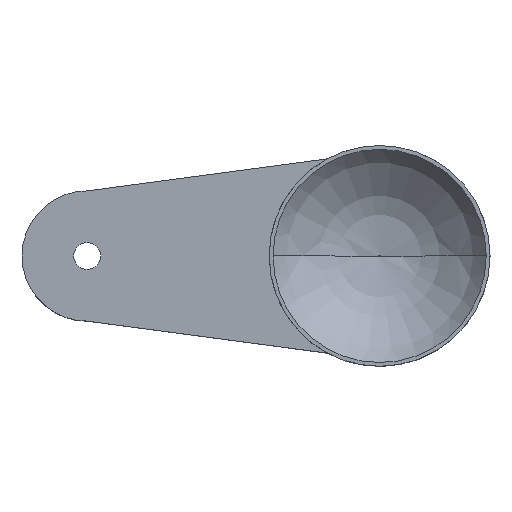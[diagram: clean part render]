
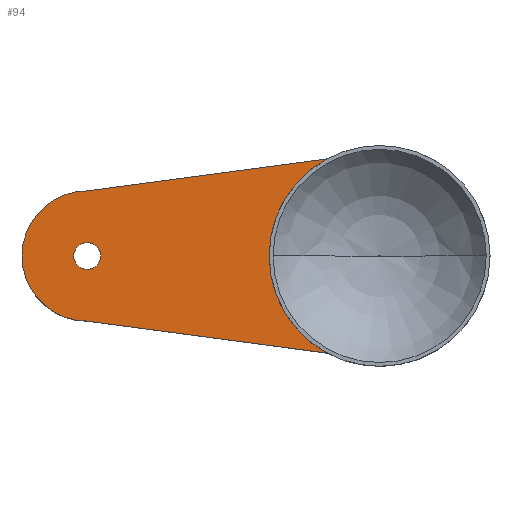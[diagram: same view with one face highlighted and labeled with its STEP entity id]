
A CAD part, top view. The second image highlights one B-rep face of the part: STEP entity #94.
In plain terms, the highlighted planar face has unit normal (0, 0, 1).
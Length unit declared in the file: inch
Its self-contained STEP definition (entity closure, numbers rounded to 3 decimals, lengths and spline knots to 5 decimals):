
#6 = LINE ( 'NONE', #535, #542 ) ;
#8 = EDGE_CURVE ( 'NONE', #490, #29, #429, .T. ) ;
#10 = DIRECTION ( 'NONE',  ( 0.991, 0.132, 0. ) ) ;
#24 = AXIS2_PLACEMENT_3D ( 'NONE', #163, #158, #155 ) ;
#29 = VERTEX_POINT ( 'NONE', #306 ) ;
#41 = DIRECTION ( 'NONE',  ( 1., 0., 0. ) ) ;
#43 = DIRECTION ( 'NONE',  ( 0., 0., 1. ) ) ;
#44 = AXIS2_PLACEMENT_3D ( 'NONE', #70, #43, #41 ) ;
#49 = EDGE_CURVE ( 'NONE', #430, #426, #289, .T. ) ;
#59 = ORIENTED_EDGE ( 'NONE', *, *, #267, .T. ) ;
#63 = CARTESIAN_POINT ( 'NONE',  ( 23.73897, 25.66022, 4. ) ) ;
#64 = CIRCLE ( 'NONE', #520, 2.43417 ) ;
#67 = CARTESIAN_POINT ( 'NONE',  ( -3.38477, 25.38511, 4. ) ) ;
#70 = CARTESIAN_POINT ( 'NONE',  ( 16.93431, 25.66022, 4. ) ) ;
#77 = ORIENTED_EDGE ( 'NONE', *, *, #460, .F. ) ;
#82 = DIRECTION ( 'NONE',  ( 1., 0., 0. ) ) ;
#85 = VECTOR ( 'NONE', #10, 39.37008 ) ;
#94 = ADVANCED_FACE ( 'NONE', ( #146, #557 ), #541, .T. ) ;
#99 = ORIENTED_EDGE ( 'NONE', *, *, #493, .F. ) ;
#146 = FACE_OUTER_BOUND ( 'NONE', #414, .T. ) ;
#155 = DIRECTION ( 'NONE',  ( 1., 0., 0. ) ) ;
#158 = DIRECTION ( 'NONE',  ( 0., 0., 1. ) ) ;
#160 = CARTESIAN_POINT ( 'NONE',  ( 16.93431, 23.22605, 4. ) ) ;
#163 = CARTESIAN_POINT ( 'NONE',  ( 27.86307, 25.66022, 4. ) ) ;
#171 = DIRECTION ( 'NONE',  ( 0., 0., 1. ) ) ;
#180 = CARTESIAN_POINT ( 'NONE',  ( 16.93431, 25.66022, 4. ) ) ;
#182 = EDGE_CURVE ( 'NONE', #317, #29, #6, .T. ) ;
#214 = ORIENTED_EDGE ( 'NONE', *, *, #539, .F. ) ;
#219 = LINE ( 'NONE', #67, #85 ) ;
#224 = DIRECTION ( 'NONE',  ( 0., 0., 1. ) ) ;
#229 = ORIENTED_EDGE ( 'NONE', *, *, #547, .T. ) ;
#260 = CARTESIAN_POINT ( 'NONE',  ( 25.90666, 29.29074, 4. ) ) ;
#267 = EDGE_CURVE ( 'NONE', #583, #317, #563, .T. ) ;
#289 = CIRCLE ( 'NONE', #417, 0.50198 ) ;
#306 = CARTESIAN_POINT ( 'NONE',  ( 25.90666, 22.0297, 4. ) ) ;
#317 = VERTEX_POINT ( 'NONE', #160 ) ;
#318 = CARTESIAN_POINT ( 'NONE',  ( 17.43629, 25.66022, 4. ) ) ;
#326 = AXIS2_PLACEMENT_3D ( 'NONE', #498, #560, #452 ) ;
#334 = ORIENTED_EDGE ( 'NONE', *, *, #182, .T. ) ;
#351 = VERTEX_POINT ( 'NONE', #260 ) ;
#399 = VERTEX_POINT ( 'NONE', #527 ) ;
#414 = EDGE_LOOP ( 'NONE', ( #99, #229, #59, #334, #606, #77 ) ) ;
#417 = AXIS2_PLACEMENT_3D ( 'NONE', #653, #650, #649 ) ;
#426 = VERTEX_POINT ( 'NONE', #489 ) ;
#429 = CIRCLE ( 'NONE', #445, 4.1241 ) ;
#430 = VERTEX_POINT ( 'NONE', #318 ) ;
#445 = AXIS2_PLACEMENT_3D ( 'NONE', #631, #224, #637 ) ;
#452 = DIRECTION ( 'NONE',  ( 1., 0., 0. ) ) ;
#454 = ORIENTED_EDGE ( 'NONE', *, *, #49, .F. ) ;
#460 = EDGE_CURVE ( 'NONE', #351, #490, #599, .T. ) ;
#468 = CIRCLE ( 'NONE', #524, 0.50198 ) ;
#489 = CARTESIAN_POINT ( 'NONE',  ( 16.43233, 25.66022, 4. ) ) ;
#490 = VERTEX_POINT ( 'NONE', #63 ) ;
#493 = EDGE_CURVE ( 'NONE', #399, #351, #219, .T. ) ;
#497 = CARTESIAN_POINT ( 'NONE',  ( 14.50013, 25.66022, 4. ) ) ;
#498 = CARTESIAN_POINT ( 'NONE',  ( 0., 0., 4. ) ) ;
#501 = DIRECTION ( 'NONE',  ( 0.991, -0.132, 0. ) ) ;
#520 = AXIS2_PLACEMENT_3D ( 'NONE', #639, #636, #630 ) ;
#524 = AXIS2_PLACEMENT_3D ( 'NONE', #180, #171, #82 ) ;
#527 = CARTESIAN_POINT ( 'NONE',  ( 16.93431, 28.09439, 4. ) ) ;
#535 = CARTESIAN_POINT ( 'NONE',  ( 3.3386, 25.03885, 4. ) ) ;
#539 = EDGE_CURVE ( 'NONE', #426, #430, #468, .T. ) ;
#541 = PLANE ( 'NONE',  #326 ) ;
#542 = VECTOR ( 'NONE', #501, 39.37008 ) ;
#547 = EDGE_CURVE ( 'NONE', #399, #583, #64, .T. ) ;
#557 = FACE_BOUND ( 'NONE', #594, .T. ) ;
#560 = DIRECTION ( 'NONE',  ( 0., 0., 1. ) ) ;
#563 = CIRCLE ( 'NONE', #44, 2.43417 ) ;
#583 = VERTEX_POINT ( 'NONE', #497 ) ;
#594 = EDGE_LOOP ( 'NONE', ( #214, #454 ) ) ;
#599 = CIRCLE ( 'NONE', #24, 4.1241 ) ;
#606 = ORIENTED_EDGE ( 'NONE', *, *, #8, .F. ) ;
#630 = DIRECTION ( 'NONE',  ( 1., 0., 0. ) ) ;
#631 = CARTESIAN_POINT ( 'NONE',  ( 27.86307, 25.66022, 4. ) ) ;
#636 = DIRECTION ( 'NONE',  ( 0., 0., 1. ) ) ;
#637 = DIRECTION ( 'NONE',  ( 1., 0., 0. ) ) ;
#639 = CARTESIAN_POINT ( 'NONE',  ( 16.93431, 25.66022, 4. ) ) ;
#649 = DIRECTION ( 'NONE',  ( 1., 0., 0. ) ) ;
#650 = DIRECTION ( 'NONE',  ( 0., 0., 1. ) ) ;
#653 = CARTESIAN_POINT ( 'NONE',  ( 16.93431, 25.66022, 4. ) ) ;
